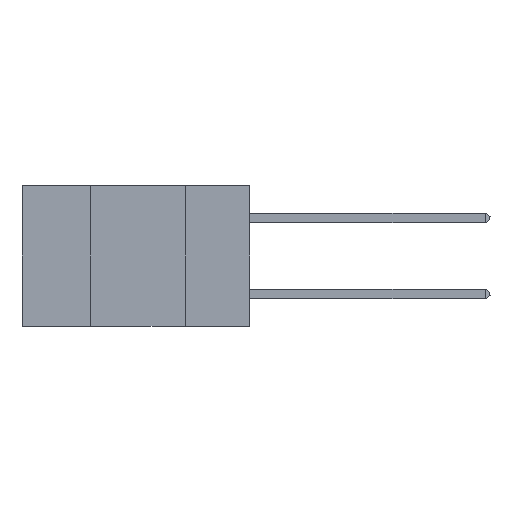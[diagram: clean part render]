
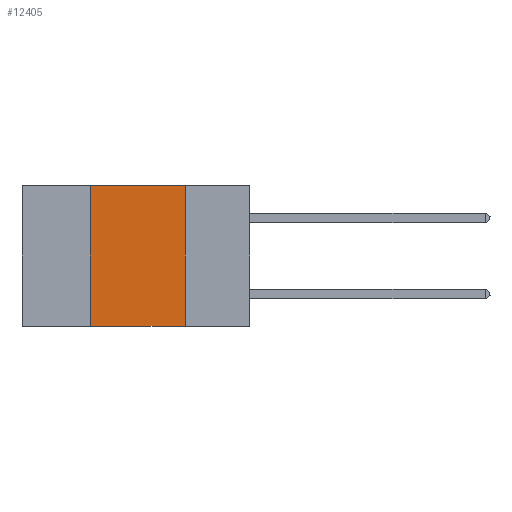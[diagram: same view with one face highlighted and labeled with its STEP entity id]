
A CAD part, left-side view. The second image highlights one B-rep face of the part: STEP entity #12405.
In plain terms, the highlighted planar face has unit normal (-1, 0, 0).
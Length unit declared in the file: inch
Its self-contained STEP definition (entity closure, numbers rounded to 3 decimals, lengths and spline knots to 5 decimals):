
#242 = EDGE_CURVE ( 'NONE', #8846, #1344, #4692, .T. ) ;
#548 = ORIENTED_EDGE ( 'NONE', *, *, #9575, .F. ) ;
#972 = DIRECTION ( 'NONE',  ( 0., 0., 1. ) ) ;
#1077 = EDGE_CURVE ( 'NONE', #5489, #13187, #15403, .T. ) ;
#1344 = VERTEX_POINT ( 'NONE', #11474 ) ;
#1360 = DIRECTION ( 'NONE',  ( 0., 0., -1. ) ) ;
#2987 = CARTESIAN_POINT ( 'NONE',  ( 0., 0.42, 0. ) ) ;
#3267 = LINE ( 'NONE', #2987, #17158 ) ;
#3526 = ORIENTED_EDGE ( 'NONE', *, *, #1077, .T. ) ;
#4692 = LINE ( 'NONE', #12793, #15007 ) ;
#4814 = DIRECTION ( 'NONE',  ( 0., -1., 0. ) ) ;
#5489 = VERTEX_POINT ( 'NONE', #17397 ) ;
#5838 = CARTESIAN_POINT ( 'NONE',  ( 0., 0.42, 0. ) ) ;
#6574 = CARTESIAN_POINT ( 'NONE',  ( 0., 0.6, -0.37 ) ) ;
#7208 = FACE_OUTER_BOUND ( 'NONE', #17314, .T. ) ;
#7502 = LINE ( 'NONE', #16965, #16359 ) ;
#8846 = VERTEX_POINT ( 'NONE', #5838 ) ;
#9575 = EDGE_CURVE ( 'NONE', #1344, #13187, #7502, .T. ) ;
#9603 = CARTESIAN_POINT ( 'NONE',  ( 0., 0.17, -0.37 ) ) ;
#9998 = ORIENTED_EDGE ( 'NONE', *, *, #242, .F. ) ;
#10230 = EDGE_CURVE ( 'NONE', #5489, #8846, #3267, .T. ) ;
#10961 = AXIS2_PLACEMENT_3D ( 'NONE', #11995, #11935, #1360 ) ;
#11220 = ORIENTED_EDGE ( 'NONE', *, *, #10230, .F. ) ;
#11371 = VECTOR ( 'NONE', #14749, 39.37008 ) ;
#11474 = CARTESIAN_POINT ( 'NONE',  ( 0., 0.17, 0. ) ) ;
#11935 = DIRECTION ( 'NONE',  ( 1., 0., 0. ) ) ;
#11995 = CARTESIAN_POINT ( 'NONE',  ( 0., 0.6, 0. ) ) ;
#12405 = ADVANCED_FACE ( 'NONE', ( #7208 ), #14604, .F. ) ;
#12793 = CARTESIAN_POINT ( 'NONE',  ( 0., 0.6, 0. ) ) ;
#12856 = DIRECTION ( 'NONE',  ( 0., 0., -1. ) ) ;
#13187 = VERTEX_POINT ( 'NONE', #9603 ) ;
#14604 = PLANE ( 'NONE',  #10961 ) ;
#14749 = DIRECTION ( 'NONE',  ( 0., -1., 0. ) ) ;
#15007 = VECTOR ( 'NONE', #4814, 39.37008 ) ;
#15403 = LINE ( 'NONE', #6574, #11371 ) ;
#16359 = VECTOR ( 'NONE', #12856, 39.37008 ) ;
#16965 = CARTESIAN_POINT ( 'NONE',  ( 0., 0.17, 0. ) ) ;
#17158 = VECTOR ( 'NONE', #972, 39.37008 ) ;
#17314 = EDGE_LOOP ( 'NONE', ( #548, #9998, #11220, #3526 ) ) ;
#17397 = CARTESIAN_POINT ( 'NONE',  ( 0., 0.42, -0.37 ) ) ;
